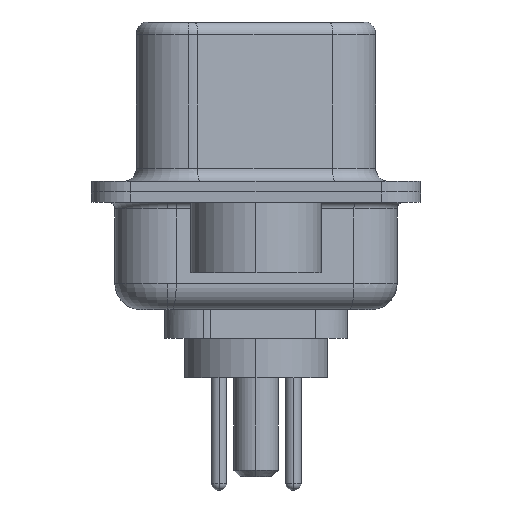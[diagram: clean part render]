
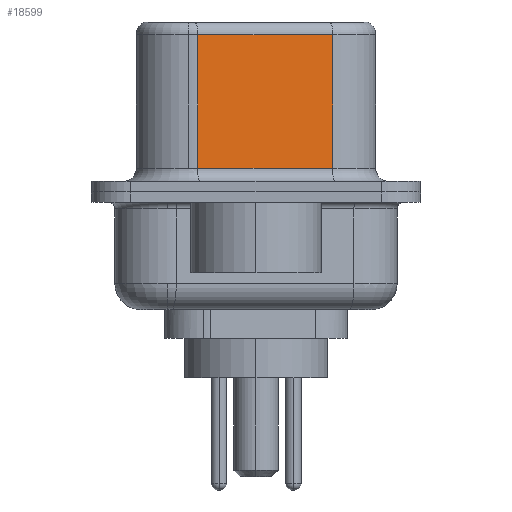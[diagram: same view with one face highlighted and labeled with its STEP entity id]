
A CAD part, left-side view. The second image highlights one B-rep face of the part: STEP entity #18599.
In plain terms, the highlighted planar face has unit normal (-0.985, -0.174, 0).
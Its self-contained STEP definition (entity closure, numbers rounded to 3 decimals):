
#221 = VECTOR ( 'NONE', #8994, 1000. ) ;
#410 = EDGE_CURVE ( 'NONE', #10434, #978, #17855, .T. ) ;
#978 = VERTEX_POINT ( 'NONE', #4378 ) ;
#1734 = CARTESIAN_POINT ( 'NONE',  ( 4.585, -2.927, 6.02 ) ) ;
#1976 = VERTEX_POINT ( 'NONE', #5515 ) ;
#2895 = EDGE_CURVE ( 'NONE', #978, #10815, #11679, .T. ) ;
#2987 = VECTOR ( 'NONE', #6860, 1000. ) ;
#3115 = EDGE_CURVE ( 'NONE', #10434, #1976, #8773, .T. ) ;
#4378 = CARTESIAN_POINT ( 'NONE',  ( 3.675, 2.233, 6.02 ) ) ;
#4978 = VECTOR ( 'NONE', #15467, 1000. ) ;
#5008 = EDGE_CURVE ( 'NONE', #10815, #1976, #6592, .T. ) ;
#5515 = CARTESIAN_POINT ( 'NONE',  ( 4.585, -2.927, 0.9 ) ) ;
#5747 = PLANE ( 'NONE',  #8938 ) ;
#6592 = LINE ( 'NONE', #9388, #2987 ) ;
#6860 = DIRECTION ( 'NONE',  ( 0.174, -0.985, 0. ) ) ;
#7118 = VECTOR ( 'NONE', #14755, 1000. ) ;
#8742 = ORIENTED_EDGE ( 'NONE', *, *, #3115, .F. ) ;
#8773 = LINE ( 'NONE', #15343, #221 ) ;
#8858 = DIRECTION ( 'NONE',  ( -0.174, 0.985, 0. ) ) ;
#8938 = AXIS2_PLACEMENT_3D ( 'NONE', #16562, #18167, #8858 ) ;
#8994 = DIRECTION ( 'NONE',  ( 0., 0., -1. ) ) ;
#9388 = CARTESIAN_POINT ( 'NONE',  ( 4.585, -2.927, 0.9 ) ) ;
#10434 = VERTEX_POINT ( 'NONE', #1734 ) ;
#10448 = CARTESIAN_POINT ( 'NONE',  ( 3.675, 2.233, 0.9 ) ) ;
#10815 = VERTEX_POINT ( 'NONE', #10448 ) ;
#11679 = LINE ( 'NONE', #14751, #7118 ) ;
#13182 = EDGE_LOOP ( 'NONE', ( #8742, #15074, #13865, #15345 ) ) ;
#13285 = FACE_OUTER_BOUND ( 'NONE', #13182, .T. ) ;
#13865 = ORIENTED_EDGE ( 'NONE', *, *, #2895, .T. ) ;
#14751 = CARTESIAN_POINT ( 'NONE',  ( 3.675, 2.233, 6.52 ) ) ;
#14755 = DIRECTION ( 'NONE',  ( 0., 0., -1. ) ) ;
#15074 = ORIENTED_EDGE ( 'NONE', *, *, #410, .T. ) ;
#15330 = CARTESIAN_POINT ( 'NONE',  ( 4.585, -2.927, 6.02 ) ) ;
#15343 = CARTESIAN_POINT ( 'NONE',  ( 4.585, -2.927, 6.52 ) ) ;
#15345 = ORIENTED_EDGE ( 'NONE', *, *, #5008, .T. ) ;
#15467 = DIRECTION ( 'NONE',  ( -0.174, 0.985, 0. ) ) ;
#16562 = CARTESIAN_POINT ( 'NONE',  ( 4.585, -2.927, 6.52 ) ) ;
#17855 = LINE ( 'NONE', #15330, #4978 ) ;
#18167 = DIRECTION ( 'NONE',  ( 0.985, 0.174, 0. ) ) ;
#18599 = ADVANCED_FACE ( 'NONE', ( #13285 ), #5747, .F. ) ;
